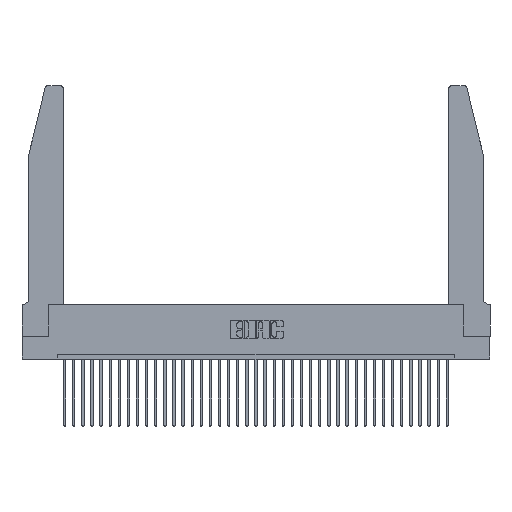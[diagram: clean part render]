
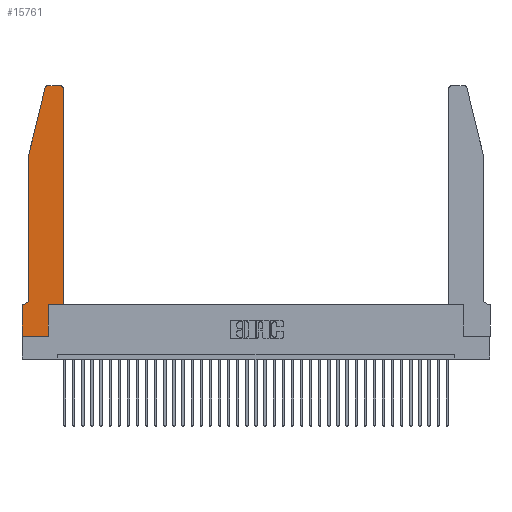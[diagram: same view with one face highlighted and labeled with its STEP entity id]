
A CAD part, top view. The second image highlights one B-rep face of the part: STEP entity #15761.
In plain terms, the highlighted planar face has unit normal (0, 0, 1).
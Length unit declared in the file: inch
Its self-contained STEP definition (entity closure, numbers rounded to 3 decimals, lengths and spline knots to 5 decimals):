
#38 = VERTEX_POINT ( 'NONE', #18632 ) ;
#797 = VECTOR ( 'NONE', #17168, 39.37008 ) ;
#1055 = PLANE ( 'NONE',  #36558 ) ;
#1154 = EDGE_CURVE ( 'NONE', #28945, #33142, #3660, .T. ) ;
#2125 = FACE_OUTER_BOUND ( 'NONE', #15794, .T. ) ;
#2268 = LINE ( 'NONE', #25531, #11177 ) ;
#2411 = VECTOR ( 'NONE', #13439, 39.37008 ) ;
#3477 = CARTESIAN_POINT ( 'NONE',  ( 0.2865, 0., 0.37 ) ) ;
#3535 = VECTOR ( 'NONE', #3854, 39.37008 ) ;
#3660 = LINE ( 'NONE', #34712, #8155 ) ;
#3854 = DIRECTION ( 'NONE',  ( 0., 1., 0. ) ) ;
#4887 = CARTESIAN_POINT ( 'NONE',  ( 0.284, 2.72, 0.37 ) ) ;
#5155 = VERTEX_POINT ( 'NONE', #30196 ) ;
#6398 = CARTESIAN_POINT ( 'NONE',  ( 0.0755, 2., 0.37 ) ) ;
#7122 = CARTESIAN_POINT ( 'NONE',  ( 0.2865, 0.35, 0.37 ) ) ;
#8011 = LINE ( 'NONE', #19140, #30343 ) ;
#8155 = VECTOR ( 'NONE', #11963, 39.37008 ) ;
#8413 = CARTESIAN_POINT ( 'NONE',  ( 0., 0., 0.37 ) ) ;
#8440 = LINE ( 'NONE', #15204, #3535 ) ;
#9039 = EDGE_CURVE ( 'NONE', #38, #19329, #9557, .T. ) ;
#9358 = DIRECTION ( 'NONE',  ( -0.239, -0.971, 0. ) ) ;
#9557 = LINE ( 'NONE', #24631, #2411 ) ;
#10926 = EDGE_CURVE ( 'NONE', #29615, #11267, #2268, .T. ) ;
#11148 = CARTESIAN_POINT ( 'NONE',  ( 0.25487, 2.72718, 0.37 ) ) ;
#11177 = VECTOR ( 'NONE', #9358, 39.37008 ) ;
#11233 = CIRCLE ( 'NONE', #24285, 0.03 ) ;
#11267 = VERTEX_POINT ( 'NONE', #13070 ) ;
#11281 = DIRECTION ( 'NONE',  ( -1., 0., 0. ) ) ;
#11833 = CARTESIAN_POINT ( 'NONE',  ( 0.4205, 2.75, 0.37 ) ) ;
#11963 = DIRECTION ( 'NONE',  ( 0., 1., 0. ) ) ;
#12235 = ORIENTED_EDGE ( 'NONE', *, *, #35269, .T. ) ;
#12293 = LINE ( 'NONE', #33769, #28309 ) ;
#12363 = AXIS2_PLACEMENT_3D ( 'NONE', #4887, #27656, #19368 ) ;
#13045 = DIRECTION ( 'NONE',  ( 0., 0., 1. ) ) ;
#13070 = CARTESIAN_POINT ( 'NONE',  ( 0.0755, 2., 0.37 ) ) ;
#13308 = CARTESIAN_POINT ( 'NONE',  ( 0., 0., 0.37 ) ) ;
#13439 = DIRECTION ( 'NONE',  ( 0., -1., 0. ) ) ;
#13556 = LINE ( 'NONE', #8413, #23283 ) ;
#15204 = CARTESIAN_POINT ( 'NONE',  ( 0.4505, 0.35, 0.37 ) ) ;
#15516 = CIRCLE ( 'NONE', #28770, 0.07 ) ;
#15534 = EDGE_CURVE ( 'NONE', #5155, #26751, #15516, .T. ) ;
#15761 = ADVANCED_FACE ( 'NONE', ( #2125 ), #1055, .T. ) ;
#15794 = EDGE_LOOP ( 'NONE', ( #12235, #31839, #27875, #29744, #31438, #32240, #16471, #18462, #34381, #32708, #30519, #28266 ) ) ;
#16169 = CARTESIAN_POINT ( 'NONE',  ( 0.4205, 2.72, 0.37 ) ) ;
#16471 = ORIENTED_EDGE ( 'NONE', *, *, #9039, .T. ) ;
#16564 = CARTESIAN_POINT ( 'NONE',  ( 0.0055, 0.42, 0.37 ) ) ;
#16569 = VERTEX_POINT ( 'NONE', #31826 ) ;
#16691 = DIRECTION ( 'NONE',  ( 1., 0., 0. ) ) ;
#17168 = DIRECTION ( 'NONE',  ( 1., 0., 0. ) ) ;
#17648 = DIRECTION ( 'NONE',  ( 1., 0., 0. ) ) ;
#17925 = EDGE_CURVE ( 'NONE', #19329, #28945, #13556, .T. ) ;
#18462 = ORIENTED_EDGE ( 'NONE', *, *, #17925, .T. ) ;
#18632 = CARTESIAN_POINT ( 'NONE',  ( 0., 0.35, 0.37 ) ) ;
#18674 = EDGE_CURVE ( 'NONE', #35050, #24505, #11233, .T. ) ;
#19140 = CARTESIAN_POINT ( 'NONE',  ( 0.2605, 2.75, 0.37 ) ) ;
#19314 = DIRECTION ( 'NONE',  ( -1., 0., 0. ) ) ;
#19329 = VERTEX_POINT ( 'NONE', #13308 ) ;
#19368 = DIRECTION ( 'NONE',  ( 1., 0., 0. ) ) ;
#20622 = EDGE_CURVE ( 'NONE', #16569, #35050, #8440, .T. ) ;
#21267 = EDGE_CURVE ( 'NONE', #33142, #16569, #35225, .T. ) ;
#21419 = DIRECTION ( 'NONE',  ( 1., 0., 0. ) ) ;
#21740 = CIRCLE ( 'NONE', #12363, 0.03 ) ;
#22701 = VECTOR ( 'NONE', #35390, 39.37008 ) ;
#23283 = VECTOR ( 'NONE', #16691, 39.37008 ) ;
#24285 = AXIS2_PLACEMENT_3D ( 'NONE', #16169, #13045, #21419 ) ;
#24394 = CARTESIAN_POINT ( 'NONE',  ( 0.284, 2.75, 0.37 ) ) ;
#24505 = VERTEX_POINT ( 'NONE', #11833 ) ;
#24631 = CARTESIAN_POINT ( 'NONE',  ( 0., 0., 0.37 ) ) ;
#25531 = CARTESIAN_POINT ( 'NONE',  ( 0.0755, 2., 0.37 ) ) ;
#26236 = LINE ( 'NONE', #6398, #22701 ) ;
#26751 = VERTEX_POINT ( 'NONE', #32597 ) ;
#27223 = VERTEX_POINT ( 'NONE', #24394 ) ;
#27656 = DIRECTION ( 'NONE',  ( 0., 0., 1. ) ) ;
#27875 = ORIENTED_EDGE ( 'NONE', *, *, #10926, .T. ) ;
#28266 = ORIENTED_EDGE ( 'NONE', *, *, #18674, .T. ) ;
#28269 = EDGE_CURVE ( 'NONE', #26751, #38, #12293, .T. ) ;
#28309 = VECTOR ( 'NONE', #11281, 39.37008 ) ;
#28770 = AXIS2_PLACEMENT_3D ( 'NONE', #16564, #36438, #19314 ) ;
#28914 = CARTESIAN_POINT ( 'NONE',  ( 0., 0.35, 0.37 ) ) ;
#28945 = VERTEX_POINT ( 'NONE', #3477 ) ;
#29615 = VERTEX_POINT ( 'NONE', #11148 ) ;
#29744 = ORIENTED_EDGE ( 'NONE', *, *, #31640, .T. ) ;
#30196 = CARTESIAN_POINT ( 'NONE',  ( 0.0755, 0.42, 0.37 ) ) ;
#30343 = VECTOR ( 'NONE', #34638, 39.37008 ) ;
#30519 = ORIENTED_EDGE ( 'NONE', *, *, #20622, .T. ) ;
#31354 = CARTESIAN_POINT ( 'NONE',  ( 0.4505, 0.35, 0.37 ) ) ;
#31438 = ORIENTED_EDGE ( 'NONE', *, *, #15534, .T. ) ;
#31640 = EDGE_CURVE ( 'NONE', #11267, #5155, #26236, .T. ) ;
#31826 = CARTESIAN_POINT ( 'NONE',  ( 0.4505, 0.35, 0.37 ) ) ;
#31839 = ORIENTED_EDGE ( 'NONE', *, *, #32747, .T. ) ;
#32240 = ORIENTED_EDGE ( 'NONE', *, *, #28269, .T. ) ;
#32597 = CARTESIAN_POINT ( 'NONE',  ( 0.0055, 0.35, 0.37 ) ) ;
#32708 = ORIENTED_EDGE ( 'NONE', *, *, #21267, .T. ) ;
#32747 = EDGE_CURVE ( 'NONE', #27223, #29615, #21740, .T. ) ;
#33142 = VERTEX_POINT ( 'NONE', #7122 ) ;
#33769 = CARTESIAN_POINT ( 'NONE',  ( 0.0755, 0.35, 0.37 ) ) ;
#34381 = ORIENTED_EDGE ( 'NONE', *, *, #1154, .T. ) ;
#34638 = DIRECTION ( 'NONE',  ( -1., 0., 0. ) ) ;
#34712 = CARTESIAN_POINT ( 'NONE',  ( 0.2865, 0.35, 0.37 ) ) ;
#34745 = DIRECTION ( 'NONE',  ( 0., 0., 1. ) ) ;
#35050 = VERTEX_POINT ( 'NONE', #35580 ) ;
#35225 = LINE ( 'NONE', #31354, #797 ) ;
#35269 = EDGE_CURVE ( 'NONE', #24505, #27223, #8011, .T. ) ;
#35390 = DIRECTION ( 'NONE',  ( 0., -1., 0. ) ) ;
#35580 = CARTESIAN_POINT ( 'NONE',  ( 0.4505, 2.72, 0.37 ) ) ;
#36438 = DIRECTION ( 'NONE',  ( 0., 0., -1. ) ) ;
#36558 = AXIS2_PLACEMENT_3D ( 'NONE', #28914, #34745, #17648 ) ;
